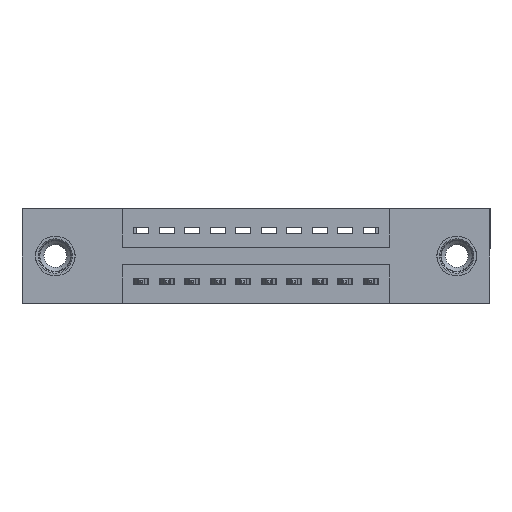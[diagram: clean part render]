
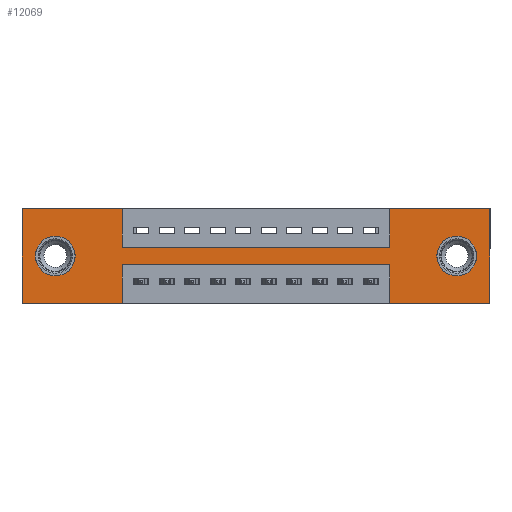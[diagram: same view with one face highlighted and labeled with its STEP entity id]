
A CAD part, front view. The second image highlights one B-rep face of the part: STEP entity #12069.
In plain terms, the highlighted planar face has unit normal (0, -1, 0).
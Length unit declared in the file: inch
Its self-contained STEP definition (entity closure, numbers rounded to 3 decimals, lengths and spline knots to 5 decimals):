
#45 = LINE ( 'NONE', #3854, #7688 ) ;
#74 = ORIENTED_EDGE ( 'NONE', *, *, #8440, .T. ) ;
#242 = VERTEX_POINT ( 'NONE', #1849 ) ;
#378 = VECTOR ( 'NONE', #14357, 39.37008 ) ;
#799 = EDGE_LOOP ( 'NONE', ( #11799, #13240 ) ) ;
#908 = AXIS2_PLACEMENT_3D ( 'NONE', #1057, #7591, #7754 ) ;
#963 = CARTESIAN_POINT ( 'NONE',  ( 1.835, 0., 0. ) ) ;
#1057 = CARTESIAN_POINT ( 'NONE',  ( 0.13, 0., -0.185 ) ) ;
#1063 = VERTEX_POINT ( 'NONE', #10305 ) ;
#1247 = LINE ( 'NONE', #13397, #6093 ) ;
#1614 = VECTOR ( 'NONE', #3717, 39.37008 ) ;
#1689 = CARTESIAN_POINT ( 'NONE',  ( 1.4425, 0., -0.37 ) ) ;
#1699 = ORIENTED_EDGE ( 'NONE', *, *, #9056, .F. ) ;
#1740 = FACE_BOUND ( 'NONE', #799, .T. ) ;
#1747 = ORIENTED_EDGE ( 'NONE', *, *, #11777, .F. ) ;
#1784 = VECTOR ( 'NONE', #10929, 39.37008 ) ;
#1849 = CARTESIAN_POINT ( 'NONE',  ( 0.13, 0., -0.107 ) ) ;
#2008 = CARTESIAN_POINT ( 'NONE',  ( 1.705, 0., -0.185 ) ) ;
#2112 = EDGE_CURVE ( 'NONE', #13336, #1063, #6832, .T. ) ;
#2243 = CIRCLE ( 'NONE', #9646, 0.078 ) ;
#2265 = VERTEX_POINT ( 'NONE', #6271 ) ;
#2304 = EDGE_LOOP ( 'NONE', ( #6818, #74 ) ) ;
#2384 = CARTESIAN_POINT ( 'NONE',  ( 1.4425, 0., -0.37 ) ) ;
#2397 = VERTEX_POINT ( 'NONE', #7895 ) ;
#2519 = CARTESIAN_POINT ( 'NONE',  ( 0., 0., -0.37 ) ) ;
#2700 = VECTOR ( 'NONE', #12456, 39.37008 ) ;
#2767 = DIRECTION ( 'NONE',  ( 0., 1., 0. ) ) ;
#2866 = CARTESIAN_POINT ( 'NONE',  ( 0., 0., 0. ) ) ;
#3142 = EDGE_CURVE ( 'NONE', #11489, #8944, #14238, .T. ) ;
#3717 = DIRECTION ( 'NONE',  ( 0., 0., -1. ) ) ;
#3777 = CARTESIAN_POINT ( 'NONE',  ( 1.705, 0., -0.263 ) ) ;
#3854 = CARTESIAN_POINT ( 'NONE',  ( 0., 0., 0. ) ) ;
#4218 = DIRECTION ( 'NONE',  ( 0., 1., 0. ) ) ;
#4353 = ORIENTED_EDGE ( 'NONE', *, *, #11387, .F. ) ;
#4428 = VERTEX_POINT ( 'NONE', #10086 ) ;
#4477 = CIRCLE ( 'NONE', #908, 0.078 ) ;
#4509 = VERTEX_POINT ( 'NONE', #2384 ) ;
#4582 = LINE ( 'NONE', #12715, #10205 ) ;
#4995 = VECTOR ( 'NONE', #5541, 39.37008 ) ;
#5055 = LINE ( 'NONE', #15279, #10705 ) ;
#5206 = EDGE_CURVE ( 'NONE', #14521, #12645, #13795, .T. ) ;
#5319 = VECTOR ( 'NONE', #14212, 39.37008 ) ;
#5468 = LINE ( 'NONE', #963, #1614 ) ;
#5490 = ORIENTED_EDGE ( 'NONE', *, *, #2112, .F. ) ;
#5541 = DIRECTION ( 'NONE',  ( 0., 0., 1. ) ) ;
#5568 = EDGE_CURVE ( 'NONE', #8802, #2397, #15580, .T. ) ;
#5617 = CARTESIAN_POINT ( 'NONE',  ( 0.3925, 0., -0.37 ) ) ;
#5707 = CARTESIAN_POINT ( 'NONE',  ( 1.4425, 0., -0.15 ) ) ;
#5991 = FACE_OUTER_BOUND ( 'NONE', #10993, .T. ) ;
#6017 = AXIS2_PLACEMENT_3D ( 'NONE', #6789, #11987, #10803 ) ;
#6093 = VECTOR ( 'NONE', #15811, 39.37008 ) ;
#6121 = CARTESIAN_POINT ( 'NONE',  ( 0.13, 0., -0.185 ) ) ;
#6271 = CARTESIAN_POINT ( 'NONE',  ( 1.835, 0., 0. ) ) ;
#6437 = ORIENTED_EDGE ( 'NONE', *, *, #12982, .F. ) ;
#6724 = CARTESIAN_POINT ( 'NONE',  ( 0.3925, 0., -0.37 ) ) ;
#6728 = LINE ( 'NONE', #15289, #5319 ) ;
#6789 = CARTESIAN_POINT ( 'NONE',  ( 0., 0., -0.37 ) ) ;
#6818 = ORIENTED_EDGE ( 'NONE', *, *, #15667, .T. ) ;
#6832 = LINE ( 'NONE', #9666, #1784 ) ;
#6856 = CARTESIAN_POINT ( 'NONE',  ( 0.3925, 0., 0. ) ) ;
#7185 = EDGE_CURVE ( 'NONE', #10320, #8802, #6728, .T. ) ;
#7318 = VERTEX_POINT ( 'NONE', #15444 ) ;
#7486 = CARTESIAN_POINT ( 'NONE',  ( 0.3925, 0., 0. ) ) ;
#7591 = DIRECTION ( 'NONE',  ( 0., 1., 0. ) ) ;
#7688 = VECTOR ( 'NONE', #12704, 39.37008 ) ;
#7705 = CARTESIAN_POINT ( 'NONE',  ( 1.835, 0., -0.37 ) ) ;
#7754 = DIRECTION ( 'NONE',  ( 0., 0., 1. ) ) ;
#7895 = CARTESIAN_POINT ( 'NONE',  ( 0.3925, 0., -0.15 ) ) ;
#7949 = ORIENTED_EDGE ( 'NONE', *, *, #16267, .F. ) ;
#8240 = CARTESIAN_POINT ( 'NONE',  ( 1.705, 0., -0.185 ) ) ;
#8319 = VERTEX_POINT ( 'NONE', #13009 ) ;
#8332 = DIRECTION ( 'NONE',  ( 0., 0., 1. ) ) ;
#8336 = ORIENTED_EDGE ( 'NONE', *, *, #3142, .F. ) ;
#8440 = EDGE_CURVE ( 'NONE', #4428, #242, #4477, .T. ) ;
#8540 = EDGE_CURVE ( 'NONE', #1063, #2265, #45, .T. ) ;
#8564 = EDGE_CURVE ( 'NONE', #8319, #11489, #1247, .T. ) ;
#8571 = DIRECTION ( 'NONE',  ( 0., 1., 0. ) ) ;
#8802 = VERTEX_POINT ( 'NONE', #6856 ) ;
#8944 = VERTEX_POINT ( 'NONE', #5617 ) ;
#9056 = EDGE_CURVE ( 'NONE', #8944, #7318, #5055, .T. ) ;
#9263 = LINE ( 'NONE', #1689, #13890 ) ;
#9453 = AXIS2_PLACEMENT_3D ( 'NONE', #2008, #4218, #14757 ) ;
#9534 = DIRECTION ( 'NONE',  ( 0., 0., -1. ) ) ;
#9587 = ORIENTED_EDGE ( 'NONE', *, *, #5568, .F. ) ;
#9646 = AXIS2_PLACEMENT_3D ( 'NONE', #6121, #8571, #15012 ) ;
#9666 = CARTESIAN_POINT ( 'NONE',  ( 1.4425, 0., 0. ) ) ;
#10032 = CIRCLE ( 'NONE', #9453, 0.078 ) ;
#10086 = CARTESIAN_POINT ( 'NONE',  ( 0.13, 0., -0.263 ) ) ;
#10205 = VECTOR ( 'NONE', #12660, 39.37008 ) ;
#10305 = CARTESIAN_POINT ( 'NONE',  ( 1.4425, 0., 0. ) ) ;
#10320 = VERTEX_POINT ( 'NONE', #13746 ) ;
#10364 = ORIENTED_EDGE ( 'NONE', *, *, #8564, .F. ) ;
#10496 = CARTESIAN_POINT ( 'NONE',  ( 1.705, 0., -0.107 ) ) ;
#10593 = CARTESIAN_POINT ( 'NONE',  ( 0.3925, 0., -0.22 ) ) ;
#10631 = ORIENTED_EDGE ( 'NONE', *, *, #16437, .F. ) ;
#10705 = VECTOR ( 'NONE', #16300, 39.37008 ) ;
#10715 = AXIS2_PLACEMENT_3D ( 'NONE', #8240, #2767, #9534 ) ;
#10803 = DIRECTION ( 'NONE',  ( 0., 0., -1. ) ) ;
#10929 = DIRECTION ( 'NONE',  ( 0., 0., 1. ) ) ;
#10993 = EDGE_LOOP ( 'NONE', ( #8336, #10364, #10631, #6437, #7949, #11741, #5490, #1747, #9587, #16186, #4353, #1699 ) ) ;
#11387 = EDGE_CURVE ( 'NONE', #7318, #10320, #13461, .T. ) ;
#11477 = EDGE_CURVE ( 'NONE', #12645, #14521, #10032, .T. ) ;
#11489 = VERTEX_POINT ( 'NONE', #10593 ) ;
#11518 = DIRECTION ( 'NONE',  ( 0., 0., -1. ) ) ;
#11741 = ORIENTED_EDGE ( 'NONE', *, *, #8540, .F. ) ;
#11777 = EDGE_CURVE ( 'NONE', #2397, #13336, #4582, .T. ) ;
#11799 = ORIENTED_EDGE ( 'NONE', *, *, #11477, .T. ) ;
#11987 = DIRECTION ( 'NONE',  ( 0., -1., 0. ) ) ;
#12069 = ADVANCED_FACE ( 'NONE', ( #1740, #12626, #5991 ), #14361, .T. ) ;
#12456 = DIRECTION ( 'NONE',  ( -1., 0., 0. ) ) ;
#12626 = FACE_BOUND ( 'NONE', #2304, .T. ) ;
#12645 = VERTEX_POINT ( 'NONE', #10496 ) ;
#12660 = DIRECTION ( 'NONE',  ( 1., 0., 0. ) ) ;
#12704 = DIRECTION ( 'NONE',  ( 1., 0., 0. ) ) ;
#12715 = CARTESIAN_POINT ( 'NONE',  ( 0.3925, 0., -0.15 ) ) ;
#12982 = EDGE_CURVE ( 'NONE', #13013, #4509, #13968, .T. ) ;
#13009 = CARTESIAN_POINT ( 'NONE',  ( 1.4425, 0., -0.22 ) ) ;
#13013 = VERTEX_POINT ( 'NONE', #7705 ) ;
#13240 = ORIENTED_EDGE ( 'NONE', *, *, #5206, .T. ) ;
#13336 = VERTEX_POINT ( 'NONE', #5707 ) ;
#13397 = CARTESIAN_POINT ( 'NONE',  ( 0.3925, 0., -0.22 ) ) ;
#13461 = LINE ( 'NONE', #2866, #4995 ) ;
#13746 = CARTESIAN_POINT ( 'NONE',  ( 0., 0., 0. ) ) ;
#13795 = CIRCLE ( 'NONE', #10715, 0.078 ) ;
#13890 = VECTOR ( 'NONE', #8332, 39.37008 ) ;
#13968 = LINE ( 'NONE', #2519, #2700 ) ;
#14212 = DIRECTION ( 'NONE',  ( 1., 0., 0. ) ) ;
#14238 = LINE ( 'NONE', #6724, #378 ) ;
#14357 = DIRECTION ( 'NONE',  ( 0., 0., -1. ) ) ;
#14361 = PLANE ( 'NONE',  #6017 ) ;
#14521 = VERTEX_POINT ( 'NONE', #3777 ) ;
#14757 = DIRECTION ( 'NONE',  ( 0., 0., -1. ) ) ;
#15012 = DIRECTION ( 'NONE',  ( 0., 0., 1. ) ) ;
#15279 = CARTESIAN_POINT ( 'NONE',  ( 0., 0., -0.37 ) ) ;
#15289 = CARTESIAN_POINT ( 'NONE',  ( 0., 0., 0. ) ) ;
#15444 = CARTESIAN_POINT ( 'NONE',  ( 0., 0., -0.37 ) ) ;
#15580 = LINE ( 'NONE', #7486, #15598 ) ;
#15598 = VECTOR ( 'NONE', #11518, 39.37008 ) ;
#15667 = EDGE_CURVE ( 'NONE', #242, #4428, #2243, .T. ) ;
#15811 = DIRECTION ( 'NONE',  ( -1., 0., 0. ) ) ;
#16186 = ORIENTED_EDGE ( 'NONE', *, *, #7185, .F. ) ;
#16267 = EDGE_CURVE ( 'NONE', #2265, #13013, #5468, .T. ) ;
#16300 = DIRECTION ( 'NONE',  ( -1., 0., 0. ) ) ;
#16437 = EDGE_CURVE ( 'NONE', #4509, #8319, #9263, .T. ) ;
